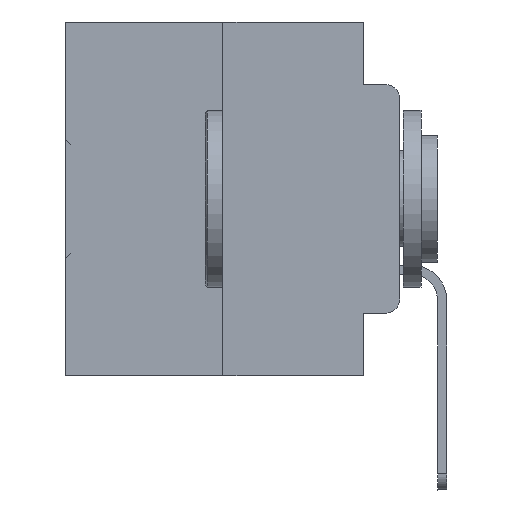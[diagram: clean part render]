
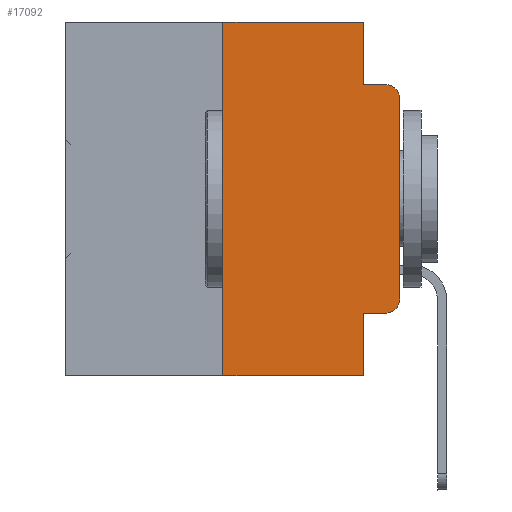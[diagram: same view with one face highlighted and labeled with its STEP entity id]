
A CAD part, left-side view. The second image highlights one B-rep face of the part: STEP entity #17092.
In plain terms, the highlighted planar face has unit normal (-1, 0, 0).
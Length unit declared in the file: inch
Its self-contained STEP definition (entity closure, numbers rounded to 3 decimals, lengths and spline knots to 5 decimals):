
#81 = CARTESIAN_POINT ( 'NONE',  ( 0., 0.25, -0.5 ) ) ;
#131 = CARTESIAN_POINT ( 'NONE',  ( 0., 0.051, -0.4115 ) ) ;
#173 = DIRECTION ( 'NONE',  ( 0., 0., -1. ) ) ;
#703 = LINE ( 'NONE', #33590, #33937 ) ;
#904 = LINE ( 'NONE', #10533, #27174 ) ;
#974 = EDGE_CURVE ( 'NONE', #7260, #26344, #13353, .T. ) ;
#1359 = PLANE ( 'NONE',  #16827 ) ;
#1929 = CARTESIAN_POINT ( 'NONE',  ( 0., 0., -0.3915 ) ) ;
#2336 = LINE ( 'NONE', #17003, #5265 ) ;
#2794 = CARTESIAN_POINT ( 'NONE',  ( 0., 0.473, 0. ) ) ;
#3094 = EDGE_LOOP ( 'NONE', ( #19357, #15229, #4503, #31767, #13538, #12103, #15787, #29101, #21421, #21804 ) ) ;
#3692 = EDGE_CURVE ( 'NONE', #27441, #29125, #20803, .T. ) ;
#4174 = VERTEX_POINT ( 'NONE', #131 ) ;
#4503 = ORIENTED_EDGE ( 'NONE', *, *, #974, .F. ) ;
#4754 = DIRECTION ( 'NONE',  ( -1., 0., 0. ) ) ;
#4800 = LINE ( 'NONE', #7469, #6217 ) ;
#5265 = VECTOR ( 'NONE', #19118, 39.37008 ) ;
#6217 = VECTOR ( 'NONE', #21230, 39.37008 ) ;
#7157 = EDGE_CURVE ( 'NONE', #4174, #12131, #10015, .T. ) ;
#7260 = VERTEX_POINT ( 'NONE', #11592 ) ;
#7363 = CARTESIAN_POINT ( 'NONE',  ( 0., 0.25, 0. ) ) ;
#7396 = VECTOR ( 'NONE', #7586, 39.37008 ) ;
#7469 = CARTESIAN_POINT ( 'NONE',  ( 0., 0.051, -0.4115 ) ) ;
#7586 = DIRECTION ( 'NONE',  ( 0., -1., 0. ) ) ;
#8589 = CARTESIAN_POINT ( 'NONE',  ( 0., 0.051, 0. ) ) ;
#9356 = DIRECTION ( 'NONE',  ( 0., -1., 0. ) ) ;
#10015 = LINE ( 'NONE', #8589, #11746 ) ;
#10533 = CARTESIAN_POINT ( 'NONE',  ( 0., 0.051, 0. ) ) ;
#10718 = DIRECTION ( 'NONE',  ( 0., 0., -1. ) ) ;
#11238 = CARTESIAN_POINT ( 'NONE',  ( 0., 0.051, -0.0885 ) ) ;
#11592 = CARTESIAN_POINT ( 'NONE',  ( 0., 0.051, -0.0885 ) ) ;
#11746 = VECTOR ( 'NONE', #32626, 39.37008 ) ;
#11771 = AXIS2_PLACEMENT_3D ( 'NONE', #24056, #19112, #173 ) ;
#12103 = ORIENTED_EDGE ( 'NONE', *, *, #13678, .F. ) ;
#12106 = CARTESIAN_POINT ( 'NONE',  ( 0., 0.051, -0.5 ) ) ;
#12118 = CARTESIAN_POINT ( 'NONE',  ( 0., 0.02, -0.0885 ) ) ;
#12131 = VERTEX_POINT ( 'NONE', #12106 ) ;
#13353 = LINE ( 'NONE', #11238, #34523 ) ;
#13538 = ORIENTED_EDGE ( 'NONE', *, *, #28023, .F. ) ;
#13678 = EDGE_CURVE ( 'NONE', #25043, #18039, #25587, .T. ) ;
#14110 = EDGE_CURVE ( 'NONE', #25043, #12131, #703, .T. ) ;
#14330 = EDGE_CURVE ( 'NONE', #15223, #26344, #18717, .T. ) ;
#14848 = DIRECTION ( 'NONE',  ( 0., 0., -1. ) ) ;
#15184 = EDGE_CURVE ( 'NONE', #4174, #27441, #4800, .T. ) ;
#15223 = VERTEX_POINT ( 'NONE', #15945 ) ;
#15229 = ORIENTED_EDGE ( 'NONE', *, *, #14330, .T. ) ;
#15787 = ORIENTED_EDGE ( 'NONE', *, *, #14110, .T. ) ;
#15945 = CARTESIAN_POINT ( 'NONE',  ( 0., 0., -0.1085 ) ) ;
#16439 = AXIS2_PLACEMENT_3D ( 'NONE', #17838, #4754, #31467 ) ;
#16827 = AXIS2_PLACEMENT_3D ( 'NONE', #16944, #33723, #14848 ) ;
#16944 = CARTESIAN_POINT ( 'NONE',  ( 0., 0.473, 0. ) ) ;
#17003 = CARTESIAN_POINT ( 'NONE',  ( 0., 0., 0. ) ) ;
#17092 = ADVANCED_FACE ( 'NONE', ( #33403 ), #1359, .F. ) ;
#17838 = CARTESIAN_POINT ( 'NONE',  ( 0., 0.02, -0.1085 ) ) ;
#17892 = CARTESIAN_POINT ( 'NONE',  ( 0., 0.02, -0.4115 ) ) ;
#18039 = VERTEX_POINT ( 'NONE', #22693 ) ;
#18304 = VERTEX_POINT ( 'NONE', #29328 ) ;
#18717 = CIRCLE ( 'NONE', #16439, 0.02 ) ;
#19112 = DIRECTION ( 'NONE',  ( -1., 0., 0. ) ) ;
#19118 = DIRECTION ( 'NONE',  ( 0., 0., 1. ) ) ;
#19357 = ORIENTED_EDGE ( 'NONE', *, *, #31687, .T. ) ;
#20803 = CIRCLE ( 'NONE', #11771, 0.02 ) ;
#21230 = DIRECTION ( 'NONE',  ( 0., -1., 0. ) ) ;
#21421 = ORIENTED_EDGE ( 'NONE', *, *, #15184, .T. ) ;
#21655 = DIRECTION ( 'NONE',  ( 0., -1., 0. ) ) ;
#21804 = ORIENTED_EDGE ( 'NONE', *, *, #3692, .T. ) ;
#21847 = EDGE_CURVE ( 'NONE', #18304, #7260, #904, .T. ) ;
#22693 = CARTESIAN_POINT ( 'NONE',  ( 0., 0.25, 0. ) ) ;
#24056 = CARTESIAN_POINT ( 'NONE',  ( 0., 0.02, -0.3915 ) ) ;
#25043 = VERTEX_POINT ( 'NONE', #81 ) ;
#25587 = LINE ( 'NONE', #7363, #34463 ) ;
#25929 = DIRECTION ( 'NONE',  ( 0., 0., 1. ) ) ;
#26344 = VERTEX_POINT ( 'NONE', #12118 ) ;
#27174 = VECTOR ( 'NONE', #10718, 39.37008 ) ;
#27441 = VERTEX_POINT ( 'NONE', #17892 ) ;
#28023 = EDGE_CURVE ( 'NONE', #18039, #18304, #34476, .T. ) ;
#29101 = ORIENTED_EDGE ( 'NONE', *, *, #7157, .F. ) ;
#29125 = VERTEX_POINT ( 'NONE', #1929 ) ;
#29328 = CARTESIAN_POINT ( 'NONE',  ( 0., 0.051, 0. ) ) ;
#31467 = DIRECTION ( 'NONE',  ( 0., 0., -1. ) ) ;
#31687 = EDGE_CURVE ( 'NONE', #29125, #15223, #2336, .T. ) ;
#31767 = ORIENTED_EDGE ( 'NONE', *, *, #21847, .F. ) ;
#32626 = DIRECTION ( 'NONE',  ( 0., 0., -1. ) ) ;
#33403 = FACE_OUTER_BOUND ( 'NONE', #3094, .T. ) ;
#33590 = CARTESIAN_POINT ( 'NONE',  ( 0., 0.473, -0.5 ) ) ;
#33723 = DIRECTION ( 'NONE',  ( 1., 0., 0. ) ) ;
#33937 = VECTOR ( 'NONE', #9356, 39.37008 ) ;
#34463 = VECTOR ( 'NONE', #25929, 39.37008 ) ;
#34476 = LINE ( 'NONE', #2794, #7396 ) ;
#34523 = VECTOR ( 'NONE', #21655, 39.37008 ) ;
